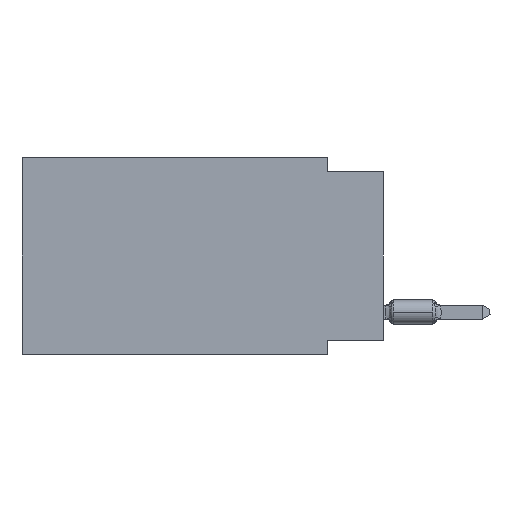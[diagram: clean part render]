
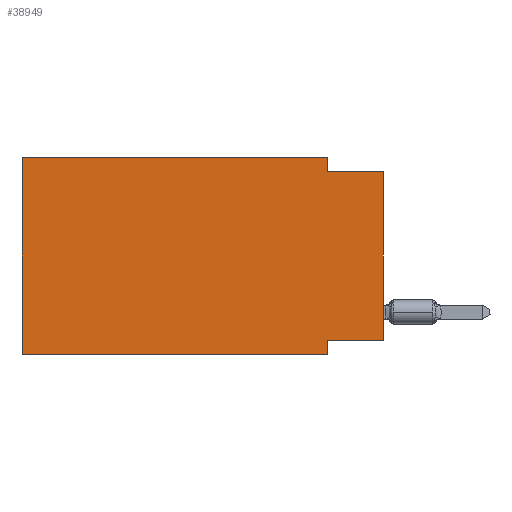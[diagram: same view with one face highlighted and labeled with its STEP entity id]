
A CAD part, left-side view. The second image highlights one B-rep face of the part: STEP entity #38949.
In plain terms, the highlighted planar face has unit normal (-1, 0, 0).
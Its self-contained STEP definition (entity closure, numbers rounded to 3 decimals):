
#129 = CARTESIAN_POINT ( 'NONE',  ( 0., 2.54, -8.255 ) ) ;
#404 = CARTESIAN_POINT ( 'NONE',  ( 0., 2.54, -8.89 ) ) ;
#1182 = ORIENTED_EDGE ( 'NONE', *, *, #68077, .F. ) ;
#1836 = CARTESIAN_POINT ( 'NONE',  ( 0., 16.383, -8.89 ) ) ;
#3003 = VERTEX_POINT ( 'NONE', #57388 ) ;
#3403 = VERTEX_POINT ( 'NONE', #63059 ) ;
#5171 = CARTESIAN_POINT ( 'NONE',  ( 0., 0., -0.635 ) ) ;
#8583 = ORIENTED_EDGE ( 'NONE', *, *, #81328, .F. ) ;
#8955 = ORIENTED_EDGE ( 'NONE', *, *, #31561, .F. ) ;
#9562 = CARTESIAN_POINT ( 'NONE',  ( 0., 16.383, 0. ) ) ;
#11977 = AXIS2_PLACEMENT_3D ( 'NONE', #76301, #45000, #46610 ) ;
#12650 = DIRECTION ( 'NONE',  ( 0., 0., 1. ) ) ;
#13080 = EDGE_CURVE ( 'NONE', #31653, #17692, #65696, .T. ) ;
#13463 = ORIENTED_EDGE ( 'NONE', *, *, #63137, .T. ) ;
#13925 = VECTOR ( 'NONE', #56612, 1000. ) ;
#14155 = LINE ( 'NONE', #58243, #13925 ) ;
#14972 = CARTESIAN_POINT ( 'NONE',  ( 0., 16.383, -8.89 ) ) ;
#15328 = VERTEX_POINT ( 'NONE', #129 ) ;
#17168 = LINE ( 'NONE', #36950, #19323 ) ;
#17586 = DIRECTION ( 'NONE',  ( 0., 1., 0. ) ) ;
#17692 = VERTEX_POINT ( 'NONE', #53022 ) ;
#17774 = EDGE_CURVE ( 'NONE', #31653, #37648, #32730, .T. ) ;
#17933 = DIRECTION ( 'NONE',  ( 0., -1., 0. ) ) ;
#18585 = EDGE_LOOP ( 'NONE', ( #13463, #59737, #8955, #48930, #68750, #20012, #1182, #8583 ) ) ;
#19323 = VECTOR ( 'NONE', #17586, 1000. ) ;
#20012 = ORIENTED_EDGE ( 'NONE', *, *, #17774, .T. ) ;
#21442 = VECTOR ( 'NONE', #64844, 1000. ) ;
#24196 = LINE ( 'NONE', #38189, #76382 ) ;
#24775 = VERTEX_POINT ( 'NONE', #51373 ) ;
#28072 = FACE_OUTER_BOUND ( 'NONE', #18585, .T. ) ;
#30312 = LINE ( 'NONE', #55447, #49259 ) ;
#31561 = EDGE_CURVE ( 'NONE', #3003, #3403, #14155, .T. ) ;
#31653 = VERTEX_POINT ( 'NONE', #14972 ) ;
#32366 = DIRECTION ( 'NONE',  ( 0., 0., -1. ) ) ;
#32730 = LINE ( 'NONE', #1836, #21442 ) ;
#34157 = VECTOR ( 'NONE', #47850, 1000. ) ;
#34406 = CARTESIAN_POINT ( 'NONE',  ( 0., 16.383, 0. ) ) ;
#36950 = CARTESIAN_POINT ( 'NONE',  ( 0., 0., -8.255 ) ) ;
#37648 = VERTEX_POINT ( 'NONE', #404 ) ;
#38189 = CARTESIAN_POINT ( 'NONE',  ( 0., 0., 0. ) ) ;
#38949 = ADVANCED_FACE ( 'NONE', ( #28072 ), #51577, .F. ) ;
#42680 = LINE ( 'NONE', #5171, #67557 ) ;
#45000 = DIRECTION ( 'NONE',  ( 1., 0., 0. ) ) ;
#46610 = DIRECTION ( 'NONE',  ( 0., 0., -1. ) ) ;
#47850 = DIRECTION ( 'NONE',  ( 0., -1., 0. ) ) ;
#48257 = EDGE_CURVE ( 'NONE', #17692, #3003, #59398, .T. ) ;
#48930 = ORIENTED_EDGE ( 'NONE', *, *, #48257, .F. ) ;
#49259 = VECTOR ( 'NONE', #32366, 1000. ) ;
#51373 = CARTESIAN_POINT ( 'NONE',  ( 0., 0., -8.255 ) ) ;
#51577 = PLANE ( 'NONE',  #11977 ) ;
#52277 = CARTESIAN_POINT ( 'NONE',  ( 0., 0., -0.635 ) ) ;
#53022 = CARTESIAN_POINT ( 'NONE',  ( 0., 16.383, 0. ) ) ;
#53650 = VECTOR ( 'NONE', #64492, 1000. ) ;
#55447 = CARTESIAN_POINT ( 'NONE',  ( 0., 2.54, -8.89 ) ) ;
#56612 = DIRECTION ( 'NONE',  ( 0., 0., -1. ) ) ;
#57388 = CARTESIAN_POINT ( 'NONE',  ( 0., 2.54, 0. ) ) ;
#58243 = CARTESIAN_POINT ( 'NONE',  ( 0., 2.54, 0. ) ) ;
#59398 = LINE ( 'NONE', #9562, #34157 ) ;
#59737 = ORIENTED_EDGE ( 'NONE', *, *, #77786, .F. ) ;
#63059 = CARTESIAN_POINT ( 'NONE',  ( 0., 2.54, -0.635 ) ) ;
#63137 = EDGE_CURVE ( 'NONE', #24775, #77062, #24196, .T. ) ;
#64492 = DIRECTION ( 'NONE',  ( 0., 0., 1. ) ) ;
#64844 = DIRECTION ( 'NONE',  ( 0., -1., 0. ) ) ;
#65696 = LINE ( 'NONE', #34406, #53650 ) ;
#67557 = VECTOR ( 'NONE', #17933, 1000. ) ;
#68077 = EDGE_CURVE ( 'NONE', #15328, #37648, #30312, .T. ) ;
#68750 = ORIENTED_EDGE ( 'NONE', *, *, #13080, .F. ) ;
#76301 = CARTESIAN_POINT ( 'NONE',  ( 0., 16.383, 0. ) ) ;
#76382 = VECTOR ( 'NONE', #12650, 1000. ) ;
#77062 = VERTEX_POINT ( 'NONE', #52277 ) ;
#77786 = EDGE_CURVE ( 'NONE', #3403, #77062, #42680, .T. ) ;
#81328 = EDGE_CURVE ( 'NONE', #24775, #15328, #17168, .T. ) ;
